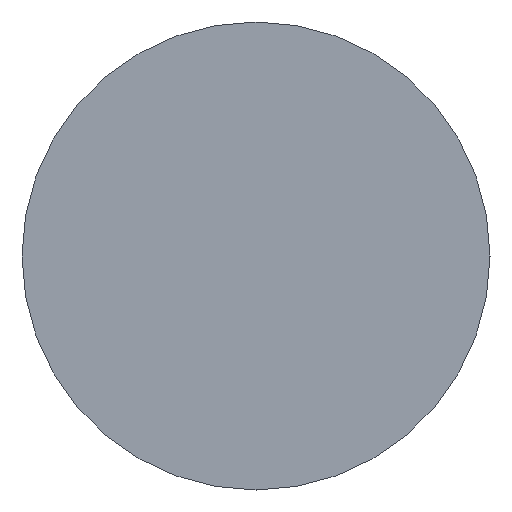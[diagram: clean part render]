
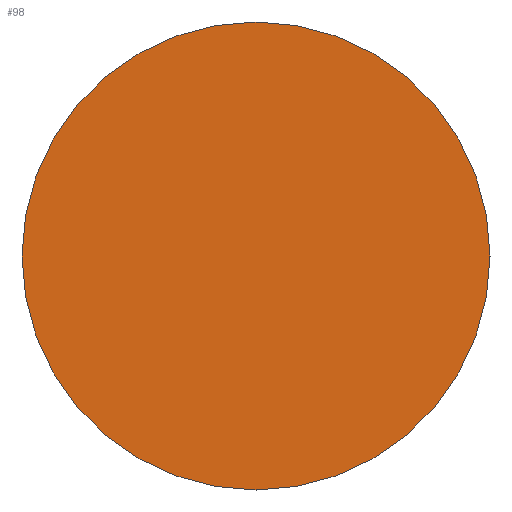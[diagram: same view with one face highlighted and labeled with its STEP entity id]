
A CAD part, front view. The second image highlights one B-rep face of the part: STEP entity #98.
In plain terms, the highlighted planar face has unit normal (0, -1, 0).
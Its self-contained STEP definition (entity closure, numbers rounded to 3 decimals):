
#8 = CIRCLE ( 'NONE', #169, 1.775 ) ;
#28 = EDGE_LOOP ( 'NONE', ( #356, #30 ) ) ;
#30 = ORIENTED_EDGE ( 'NONE', *, *, #366, .T. ) ;
#31 = FACE_OUTER_BOUND ( 'NONE', #28, .T. ) ;
#98 = ADVANCED_FACE ( 'NONE', ( #31 ), #334, .T. ) ;
#107 = DIRECTION ( 'NONE',  ( 0., 0., -1. ) ) ;
#108 = DIRECTION ( 'NONE',  ( 0., -1., 0. ) ) ;
#109 = CARTESIAN_POINT ( 'NONE',  ( 0., 0., 0. ) ) ;
#110 = DIRECTION ( 'NONE',  ( 0., 0., -1. ) ) ;
#111 = DIRECTION ( 'NONE',  ( 0., -1., 0. ) ) ;
#113 = CARTESIAN_POINT ( 'NONE',  ( 0., 0., 0. ) ) ;
#169 = AXIS2_PLACEMENT_3D ( 'NONE', #109, #108, #107 ) ;
#170 = AXIS2_PLACEMENT_3D ( 'NONE', #113, #111, #110 ) ;
#237 = CARTESIAN_POINT ( 'NONE',  ( 0., 0., -1.775 ) ) ;
#243 = CARTESIAN_POINT ( 'NONE',  ( 0., 0., 1.775 ) ) ;
#245 = AXIS2_PLACEMENT_3D ( 'NONE', #336, #339, #333 ) ;
#278 = VERTEX_POINT ( 'NONE', #243 ) ;
#288 = CIRCLE ( 'NONE', #170, 1.775 ) ;
#298 = VERTEX_POINT ( 'NONE', #237 ) ;
#333 = DIRECTION ( 'NONE',  ( 0., 0., -1. ) ) ;
#334 = PLANE ( 'NONE',  #245 ) ;
#336 = CARTESIAN_POINT ( 'NONE',  ( 0., 0., 0. ) ) ;
#339 = DIRECTION ( 'NONE',  ( 0., -1., 0. ) ) ;
#356 = ORIENTED_EDGE ( 'NONE', *, *, #361, .T. ) ;
#361 = EDGE_CURVE ( 'NONE', #298, #278, #288, .T. ) ;
#366 = EDGE_CURVE ( 'NONE', #278, #298, #8, .T. ) ;
